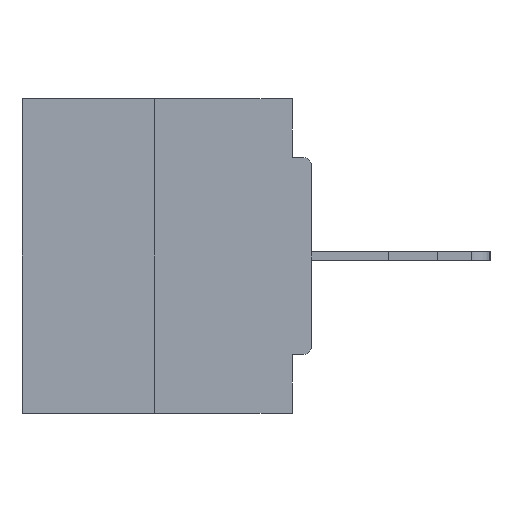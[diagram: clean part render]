
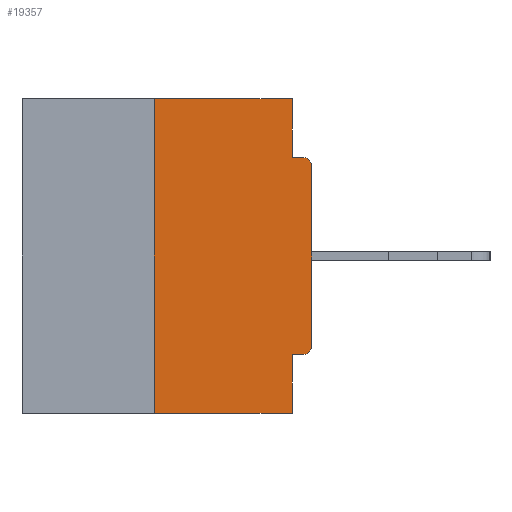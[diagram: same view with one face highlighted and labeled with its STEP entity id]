
A CAD part, left-side view. The second image highlights one B-rep face of the part: STEP entity #19357.
In plain terms, the highlighted planar face has unit normal (-1, 0, 0).
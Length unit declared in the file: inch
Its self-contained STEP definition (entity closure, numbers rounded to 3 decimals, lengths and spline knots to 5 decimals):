
#21 = EDGE_CURVE ( 'NONE', #2953, #1054, #22990, .T. ) ;
#560 = VECTOR ( 'NONE', #25149, 39.37008 ) ;
#886 = DIRECTION ( 'NONE',  ( -1., 0., 0. ) ) ;
#975 = CARTESIAN_POINT ( 'NONE',  ( 0., 0.031, 0. ) ) ;
#1054 = VERTEX_POINT ( 'NONE', #15275 ) ;
#1135 = PLANE ( 'NONE',  #19141 ) ;
#2638 = ORIENTED_EDGE ( 'NONE', *, *, #8160, .T. ) ;
#2922 = DIRECTION ( 'NONE',  ( 0., 1., 0. ) ) ;
#2931 = DIRECTION ( 'NONE',  ( 0., 0., 1. ) ) ;
#2953 = VERTEX_POINT ( 'NONE', #27693 ) ;
#3130 = VECTOR ( 'NONE', #20274, 39.37008 ) ;
#3274 = VECTOR ( 'NONE', #27640, 39.37008 ) ;
#3445 = ORIENTED_EDGE ( 'NONE', *, *, #26130, .F. ) ;
#3739 = DIRECTION ( 'NONE',  ( 1., 0., 0. ) ) ;
#3838 = CARTESIAN_POINT ( 'NONE',  ( 0., 0., 0. ) ) ;
#4281 = DIRECTION ( 'NONE',  ( -1., 0., 0. ) ) ;
#4385 = VERTEX_POINT ( 'NONE', #9981 ) ;
#5353 = EDGE_CURVE ( 'NONE', #22324, #2953, #27048, .T. ) ;
#5609 = CARTESIAN_POINT ( 'NONE',  ( 0., 0.031, -0.5 ) ) ;
#5969 = CARTESIAN_POINT ( 'NONE',  ( 0., 0.015, -0.3915 ) ) ;
#6348 = CARTESIAN_POINT ( 'NONE',  ( 0., 0.015, -0.4065 ) ) ;
#6909 = LINE ( 'NONE', #19354, #20725 ) ;
#7480 = ORIENTED_EDGE ( 'NONE', *, *, #21, .T. ) ;
#8160 = EDGE_CURVE ( 'NONE', #11861, #11190, #15099, .T. ) ;
#8566 = CARTESIAN_POINT ( 'NONE',  ( 0., 0.25, -0.5 ) ) ;
#8746 = CARTESIAN_POINT ( 'NONE',  ( 0., 0.46, 0. ) ) ;
#8876 = VERTEX_POINT ( 'NONE', #25554 ) ;
#9040 = EDGE_CURVE ( 'NONE', #11861, #4385, #22283, .T. ) ;
#9055 = VERTEX_POINT ( 'NONE', #23887 ) ;
#9095 = ORIENTED_EDGE ( 'NONE', *, *, #13872, .T. ) ;
#9618 = CARTESIAN_POINT ( 'NONE',  ( 0., 0.46, -0.5 ) ) ;
#9981 = CARTESIAN_POINT ( 'NONE',  ( 0., 0.25, 0. ) ) ;
#10021 = CARTESIAN_POINT ( 'NONE',  ( 0., 0.031, -0.0935 ) ) ;
#10363 = DIRECTION ( 'NONE',  ( 0., 0., -1. ) ) ;
#10576 = VECTOR ( 'NONE', #23771, 39.37008 ) ;
#10727 = VERTEX_POINT ( 'NONE', #975 ) ;
#11190 = VERTEX_POINT ( 'NONE', #5609 ) ;
#11861 = VERTEX_POINT ( 'NONE', #8566 ) ;
#13361 = CARTESIAN_POINT ( 'NONE',  ( 0., 0., -0.0935 ) ) ;
#13365 = CARTESIAN_POINT ( 'NONE',  ( 0., 0.25, 0. ) ) ;
#13752 = CARTESIAN_POINT ( 'NONE',  ( 0., 0.46, 0. ) ) ;
#13872 = EDGE_CURVE ( 'NONE', #1054, #8876, #18651, .T. ) ;
#13937 = EDGE_CURVE ( 'NONE', #10727, #24561, #31485, .T. ) ;
#15099 = LINE ( 'NONE', #9618, #560 ) ;
#15275 = CARTESIAN_POINT ( 'NONE',  ( 0., 0., -0.1085 ) ) ;
#15500 = EDGE_CURVE ( 'NONE', #4385, #10727, #23317, .T. ) ;
#15795 = CARTESIAN_POINT ( 'NONE',  ( 0., 0., -0.4065 ) ) ;
#18651 = CIRCLE ( 'NONE', #22280, 0.015 ) ;
#18836 = ORIENTED_EDGE ( 'NONE', *, *, #32078, .F. ) ;
#19141 = AXIS2_PLACEMENT_3D ( 'NONE', #13752, #3739, #21875 ) ;
#19354 = CARTESIAN_POINT ( 'NONE',  ( 0., 0.031, -0.5 ) ) ;
#19357 = ADVANCED_FACE ( 'NONE', ( #29069 ), #1135, .F. ) ;
#19795 = CARTESIAN_POINT ( 'NONE',  ( 0., 0.015, -0.1085 ) ) ;
#20274 = DIRECTION ( 'NONE',  ( 0., 0., 1. ) ) ;
#20725 = VECTOR ( 'NONE', #21960, 39.37008 ) ;
#21287 = EDGE_LOOP ( 'NONE', ( #28483, #22493, #2638, #3445, #18836, #32430, #7480, #9095, #22923, #31278 ) ) ;
#21478 = VECTOR ( 'NONE', #2931, 39.37008 ) ;
#21875 = DIRECTION ( 'NONE',  ( 0., 0., -1. ) ) ;
#21960 = DIRECTION ( 'NONE',  ( 0., 0., -1. ) ) ;
#22280 = AXIS2_PLACEMENT_3D ( 'NONE', #19795, #4281, #22407 ) ;
#22283 = LINE ( 'NONE', #13365, #21478 ) ;
#22324 = VERTEX_POINT ( 'NONE', #6348 ) ;
#22407 = DIRECTION ( 'NONE',  ( 0., 0., -1. ) ) ;
#22493 = ORIENTED_EDGE ( 'NONE', *, *, #9040, .F. ) ;
#22923 = ORIENTED_EDGE ( 'NONE', *, *, #30597, .F. ) ;
#22990 = LINE ( 'NONE', #3838, #3130 ) ;
#23317 = LINE ( 'NONE', #8746, #29282 ) ;
#23771 = DIRECTION ( 'NONE',  ( 0., -1., 0. ) ) ;
#23887 = CARTESIAN_POINT ( 'NONE',  ( 0., 0.031, -0.4065 ) ) ;
#24561 = VERTEX_POINT ( 'NONE', #10021 ) ;
#25149 = DIRECTION ( 'NONE',  ( 0., -1., 0. ) ) ;
#25554 = CARTESIAN_POINT ( 'NONE',  ( 0., 0.015, -0.0935 ) ) ;
#26130 = EDGE_CURVE ( 'NONE', #9055, #11190, #6909, .T. ) ;
#26717 = LINE ( 'NONE', #15795, #31855 ) ;
#27048 = CIRCLE ( 'NONE', #28304, 0.015 ) ;
#27640 = DIRECTION ( 'NONE',  ( 0., 0., -1. ) ) ;
#27693 = CARTESIAN_POINT ( 'NONE',  ( 0., 0., -0.3915 ) ) ;
#28304 = AXIS2_PLACEMENT_3D ( 'NONE', #5969, #886, #10363 ) ;
#28483 = ORIENTED_EDGE ( 'NONE', *, *, #15500, .F. ) ;
#29069 = FACE_OUTER_BOUND ( 'NONE', #21287, .T. ) ;
#29282 = VECTOR ( 'NONE', #31924, 39.37008 ) ;
#30193 = CARTESIAN_POINT ( 'NONE',  ( 0., 0.031, 0. ) ) ;
#30597 = EDGE_CURVE ( 'NONE', #24561, #8876, #31130, .T. ) ;
#31130 = LINE ( 'NONE', #13361, #10576 ) ;
#31278 = ORIENTED_EDGE ( 'NONE', *, *, #13937, .F. ) ;
#31485 = LINE ( 'NONE', #30193, #3274 ) ;
#31855 = VECTOR ( 'NONE', #2922, 39.37008 ) ;
#31924 = DIRECTION ( 'NONE',  ( 0., -1., 0. ) ) ;
#32078 = EDGE_CURVE ( 'NONE', #22324, #9055, #26717, .T. ) ;
#32430 = ORIENTED_EDGE ( 'NONE', *, *, #5353, .T. ) ;
